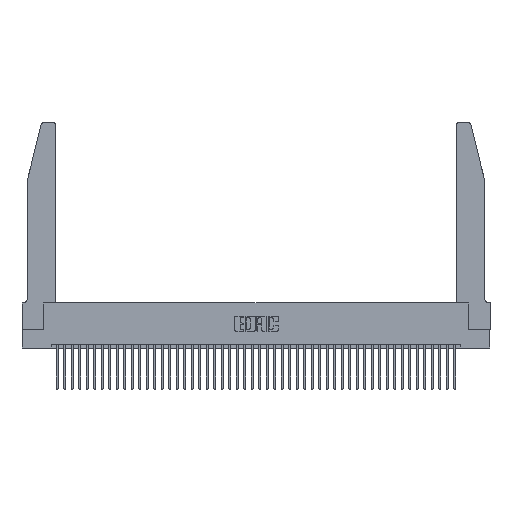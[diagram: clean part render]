
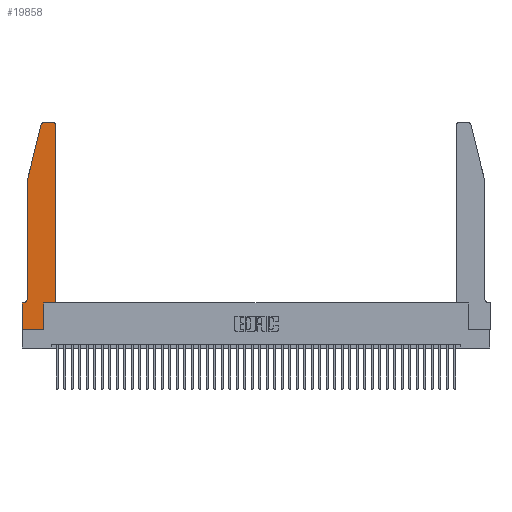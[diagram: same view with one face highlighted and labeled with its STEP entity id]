
A CAD part, top view. The second image highlights one B-rep face of the part: STEP entity #19858.
In plain terms, the highlighted planar face has unit normal (0, 0, 1).
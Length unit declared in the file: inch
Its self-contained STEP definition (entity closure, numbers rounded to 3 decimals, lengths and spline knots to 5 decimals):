
#50 = LINE ( 'NONE', #39922, #34179 ) ;
#337 = DIRECTION ( 'NONE',  ( 0., 0., 1. ) ) ;
#1094 = EDGE_CURVE ( 'NONE', #31006, #30845, #12884, .T. ) ;
#1132 = VERTEX_POINT ( 'NONE', #20862 ) ;
#1904 = VECTOR ( 'NONE', #16139, 39.37008 ) ;
#2669 = ORIENTED_EDGE ( 'NONE', *, *, #39934, .T. ) ;
#4663 = VERTEX_POINT ( 'NONE', #15573 ) ;
#5392 = EDGE_CURVE ( 'NONE', #20493, #36185, #15932, .T. ) ;
#6114 = ORIENTED_EDGE ( 'NONE', *, *, #18918, .T. ) ;
#6969 = DIRECTION ( 'NONE',  ( 1., 0., 0. ) ) ;
#7515 = EDGE_CURVE ( 'NONE', #34507, #41446, #20115, .T. ) ;
#8132 = AXIS2_PLACEMENT_3D ( 'NONE', #17856, #337, #6969 ) ;
#8575 = ORIENTED_EDGE ( 'NONE', *, *, #20821, .T. ) ;
#8584 = CARTESIAN_POINT ( 'NONE',  ( 0.2865, 0.35, 0.37 ) ) ;
#9280 = DIRECTION ( 'NONE',  ( 1., 0., 0. ) ) ;
#9911 = ORIENTED_EDGE ( 'NONE', *, *, #21989, .T. ) ;
#10739 = DIRECTION ( 'NONE',  ( 1., 0., 0. ) ) ;
#11436 = EDGE_CURVE ( 'NONE', #43859, #1132, #27192, .T. ) ;
#12276 = AXIS2_PLACEMENT_3D ( 'NONE', #15813, #26262, #36740 ) ;
#12606 = ORIENTED_EDGE ( 'NONE', *, *, #34412, .T. ) ;
#12884 = CIRCLE ( 'NONE', #28944, 0.03 ) ;
#13954 = DIRECTION ( 'NONE',  ( 0., 0., 1. ) ) ;
#14367 = VECTOR ( 'NONE', #26098, 39.37008 ) ;
#15303 = VECTOR ( 'NONE', #40108, 39.37008 ) ;
#15309 = CARTESIAN_POINT ( 'NONE',  ( 0.0055, 0.35, 0.37 ) ) ;
#15495 = CIRCLE ( 'NONE', #40604, 0.07 ) ;
#15573 = CARTESIAN_POINT ( 'NONE',  ( 0.4505, 0.35, 0.37 ) ) ;
#15725 = VECTOR ( 'NONE', #9280, 39.37008 ) ;
#15813 = CARTESIAN_POINT ( 'NONE',  ( 0.4205, 2.72, 0.37 ) ) ;
#15932 = CIRCLE ( 'NONE', #12276, 0.03 ) ;
#16139 = DIRECTION ( 'NONE',  ( 0., -1., 0. ) ) ;
#16250 = CARTESIAN_POINT ( 'NONE',  ( 0.4505, 0.35, 0.37 ) ) ;
#16544 = CARTESIAN_POINT ( 'NONE',  ( 0.2865, 0., 0.37 ) ) ;
#16563 = CARTESIAN_POINT ( 'NONE',  ( 0.0755, 0.35, 0.37 ) ) ;
#16669 = LINE ( 'NONE', #16250, #42033 ) ;
#17453 = CARTESIAN_POINT ( 'NONE',  ( 0.284, 2.72, 0.37 ) ) ;
#17856 = CARTESIAN_POINT ( 'NONE',  ( 0., 0.35, 0.37 ) ) ;
#17930 = DIRECTION ( 'NONE',  ( -1., 0., 0. ) ) ;
#18918 = EDGE_CURVE ( 'NONE', #42580, #31074, #42436, .T. ) ;
#19076 = ORIENTED_EDGE ( 'NONE', *, *, #7515, .T. ) ;
#19323 = VECTOR ( 'NONE', #44206, 39.37008 ) ;
#19557 = CARTESIAN_POINT ( 'NONE',  ( 0., 0., 0.37 ) ) ;
#19858 = ADVANCED_FACE ( 'NONE', ( #26375 ), #28304, .T. ) ;
#20112 = CARTESIAN_POINT ( 'NONE',  ( 0., 0., 0.37 ) ) ;
#20115 = LINE ( 'NONE', #19557, #15725 ) ;
#20493 = VERTEX_POINT ( 'NONE', #27508 ) ;
#20542 = ORIENTED_EDGE ( 'NONE', *, *, #24611, .T. ) ;
#20821 = EDGE_CURVE ( 'NONE', #4663, #20493, #22453, .T. ) ;
#20862 = CARTESIAN_POINT ( 'NONE',  ( 0., 0.35, 0.37 ) ) ;
#20896 = VERTEX_POINT ( 'NONE', #8584 ) ;
#21634 = EDGE_LOOP ( 'NONE', ( #9911, #24491, #20542, #6114, #12606, #44132, #30195, #19076, #2669, #45550, #8575, #36389 ) ) ;
#21989 = EDGE_CURVE ( 'NONE', #36185, #31006, #38298, .T. ) ;
#22453 = LINE ( 'NONE', #44716, #15303 ) ;
#24391 = VECTOR ( 'NONE', #40739, 39.37008 ) ;
#24491 = ORIENTED_EDGE ( 'NONE', *, *, #1094, .T. ) ;
#24611 = EDGE_CURVE ( 'NONE', #30845, #42580, #50, .T. ) ;
#25691 = CARTESIAN_POINT ( 'NONE',  ( 0., 0., 0.37 ) ) ;
#26098 = DIRECTION ( 'NONE',  ( 0., -1., 0. ) ) ;
#26262 = DIRECTION ( 'NONE',  ( 0., 0., 1. ) ) ;
#26375 = FACE_OUTER_BOUND ( 'NONE', #21634, .T. ) ;
#26720 = DIRECTION ( 'NONE',  ( 1., 0., 0. ) ) ;
#27192 = LINE ( 'NONE', #16563, #24391 ) ;
#27508 = CARTESIAN_POINT ( 'NONE',  ( 0.4505, 2.72, 0.37 ) ) ;
#28279 = CARTESIAN_POINT ( 'NONE',  ( 0.0755, 0.42, 0.37 ) ) ;
#28304 = PLANE ( 'NONE',  #8132 ) ;
#28674 = LINE ( 'NONE', #36980, #19323 ) ;
#28944 = AXIS2_PLACEMENT_3D ( 'NONE', #17453, #13954, #10739 ) ;
#30195 = ORIENTED_EDGE ( 'NONE', *, *, #32656, .T. ) ;
#30309 = DIRECTION ( 'NONE',  ( 0., 0., -1. ) ) ;
#30605 = DIRECTION ( 'NONE',  ( -1., 0., 0. ) ) ;
#30845 = VERTEX_POINT ( 'NONE', #40481 ) ;
#31006 = VERTEX_POINT ( 'NONE', #37845 ) ;
#31074 = VERTEX_POINT ( 'NONE', #28279 ) ;
#32656 = EDGE_CURVE ( 'NONE', #1132, #34507, #35497, .T. ) ;
#34179 = VECTOR ( 'NONE', #43601, 39.37008 ) ;
#34412 = EDGE_CURVE ( 'NONE', #31074, #43859, #15495, .T. ) ;
#34451 = CARTESIAN_POINT ( 'NONE',  ( 0.0055, 0.42, 0.37 ) ) ;
#34507 = VERTEX_POINT ( 'NONE', #20112 ) ;
#35485 = CARTESIAN_POINT ( 'NONE',  ( 0.2605, 2.75, 0.37 ) ) ;
#35497 = LINE ( 'NONE', #25691, #1904 ) ;
#36185 = VERTEX_POINT ( 'NONE', #44139 ) ;
#36389 = ORIENTED_EDGE ( 'NONE', *, *, #5392, .T. ) ;
#36731 = CARTESIAN_POINT ( 'NONE',  ( 0.0755, 2., 0.37 ) ) ;
#36740 = DIRECTION ( 'NONE',  ( 1., 0., 0. ) ) ;
#36980 = CARTESIAN_POINT ( 'NONE',  ( 0.2865, 0.35, 0.37 ) ) ;
#37845 = CARTESIAN_POINT ( 'NONE',  ( 0.284, 2.75, 0.37 ) ) ;
#38298 = LINE ( 'NONE', #35485, #44348 ) ;
#38622 = EDGE_CURVE ( 'NONE', #20896, #4663, #16669, .T. ) ;
#39922 = CARTESIAN_POINT ( 'NONE',  ( 0.0755, 2., 0.37 ) ) ;
#39934 = EDGE_CURVE ( 'NONE', #41446, #20896, #28674, .T. ) ;
#40108 = DIRECTION ( 'NONE',  ( 0., 1., 0. ) ) ;
#40465 = CARTESIAN_POINT ( 'NONE',  ( 0.0755, 2., 0.37 ) ) ;
#40481 = CARTESIAN_POINT ( 'NONE',  ( 0.25487, 2.72718, 0.37 ) ) ;
#40604 = AXIS2_PLACEMENT_3D ( 'NONE', #34451, #30309, #30605 ) ;
#40739 = DIRECTION ( 'NONE',  ( -1., 0., 0. ) ) ;
#41446 = VERTEX_POINT ( 'NONE', #16544 ) ;
#42033 = VECTOR ( 'NONE', #26720, 39.37008 ) ;
#42436 = LINE ( 'NONE', #36731, #14367 ) ;
#42580 = VERTEX_POINT ( 'NONE', #40465 ) ;
#43601 = DIRECTION ( 'NONE',  ( -0.239, -0.971, 0. ) ) ;
#43859 = VERTEX_POINT ( 'NONE', #15309 ) ;
#44132 = ORIENTED_EDGE ( 'NONE', *, *, #11436, .T. ) ;
#44139 = CARTESIAN_POINT ( 'NONE',  ( 0.4205, 2.75, 0.37 ) ) ;
#44206 = DIRECTION ( 'NONE',  ( 0., 1., 0. ) ) ;
#44348 = VECTOR ( 'NONE', #17930, 39.37008 ) ;
#44716 = CARTESIAN_POINT ( 'NONE',  ( 0.4505, 0.35, 0.37 ) ) ;
#45550 = ORIENTED_EDGE ( 'NONE', *, *, #38622, .T. ) ;
